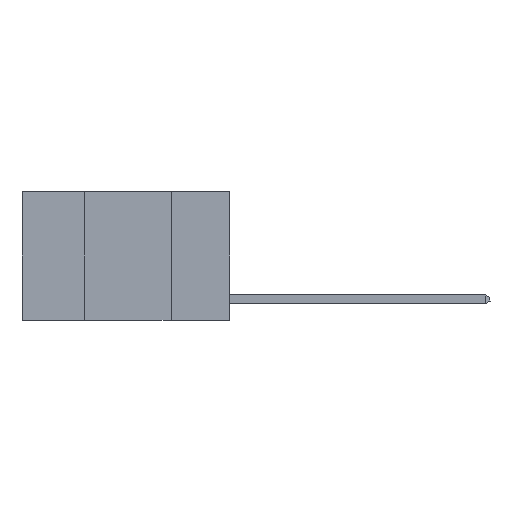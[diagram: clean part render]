
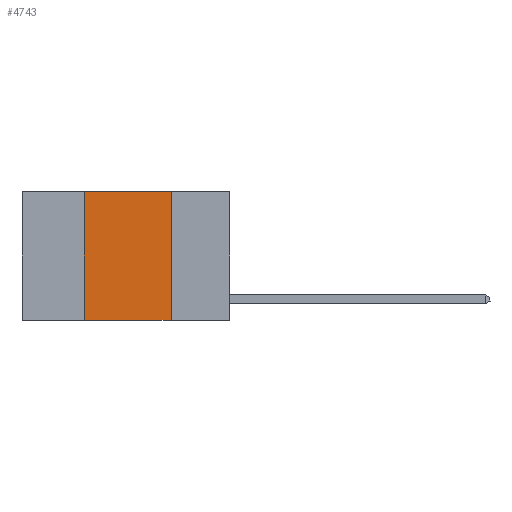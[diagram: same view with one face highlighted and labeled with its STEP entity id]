
A CAD part, left-side view. The second image highlights one B-rep face of the part: STEP entity #4743.
In plain terms, the highlighted planar face has unit normal (-1, 0, 0).
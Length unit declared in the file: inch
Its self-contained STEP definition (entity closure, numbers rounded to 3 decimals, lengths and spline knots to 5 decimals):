
#168 = PLANE ( 'NONE',  #10756 ) ;
#382 = DIRECTION ( 'NONE',  ( 0., 0., -1. ) ) ;
#2377 = ORIENTED_EDGE ( 'NONE', *, *, #10559, .F. ) ;
#3286 = VERTEX_POINT ( 'NONE', #4588 ) ;
#4561 = LINE ( 'NONE', #10851, #15903 ) ;
#4588 = CARTESIAN_POINT ( 'NONE',  ( 0., 0.17, -0.37 ) ) ;
#4635 = CARTESIAN_POINT ( 'NONE',  ( 0., 0.17, 0. ) ) ;
#4743 = ADVANCED_FACE ( 'NONE', ( #15711 ), #168, .F. ) ;
#7026 = EDGE_CURVE ( 'NONE', #7331, #3286, #4561, .T. ) ;
#7036 = LINE ( 'NONE', #19279, #10095 ) ;
#7270 = VERTEX_POINT ( 'NONE', #19467 ) ;
#7331 = VERTEX_POINT ( 'NONE', #8660 ) ;
#8660 = CARTESIAN_POINT ( 'NONE',  ( 0., 0.42, -0.37 ) ) ;
#9662 = ORIENTED_EDGE ( 'NONE', *, *, #11204, .F. ) ;
#10020 = CARTESIAN_POINT ( 'NONE',  ( 0., 0.42, 0. ) ) ;
#10095 = VECTOR ( 'NONE', #19478, 39.37008 ) ;
#10559 = EDGE_CURVE ( 'NONE', #18248, #7270, #7036, .T. ) ;
#10756 = AXIS2_PLACEMENT_3D ( 'NONE', #19101, #14469, #382 ) ;
#10851 = CARTESIAN_POINT ( 'NONE',  ( 0., 0.6, -0.37 ) ) ;
#11204 = EDGE_CURVE ( 'NONE', #7270, #3286, #18518, .T. ) ;
#11758 = VECTOR ( 'NONE', #18741, 39.37008 ) ;
#12166 = LINE ( 'NONE', #12579, #18736 ) ;
#12579 = CARTESIAN_POINT ( 'NONE',  ( 0., 0.42, 0. ) ) ;
#14469 = DIRECTION ( 'NONE',  ( 1., 0., 0. ) ) ;
#15502 = ORIENTED_EDGE ( 'NONE', *, *, #20222, .F. ) ;
#15711 = FACE_OUTER_BOUND ( 'NONE', #17831, .T. ) ;
#15903 = VECTOR ( 'NONE', #18776, 39.37008 ) ;
#16183 = ORIENTED_EDGE ( 'NONE', *, *, #7026, .T. ) ;
#17288 = DIRECTION ( 'NONE',  ( 0., 0., 1. ) ) ;
#17831 = EDGE_LOOP ( 'NONE', ( #9662, #2377, #15502, #16183 ) ) ;
#18248 = VERTEX_POINT ( 'NONE', #10020 ) ;
#18518 = LINE ( 'NONE', #4635, #11758 ) ;
#18736 = VECTOR ( 'NONE', #17288, 39.37008 ) ;
#18741 = DIRECTION ( 'NONE',  ( 0., 0., -1. ) ) ;
#18776 = DIRECTION ( 'NONE',  ( 0., -1., 0. ) ) ;
#19101 = CARTESIAN_POINT ( 'NONE',  ( 0., 0.6, 0. ) ) ;
#19279 = CARTESIAN_POINT ( 'NONE',  ( 0., 0.6, 0. ) ) ;
#19467 = CARTESIAN_POINT ( 'NONE',  ( 0., 0.17, 0. ) ) ;
#19478 = DIRECTION ( 'NONE',  ( 0., -1., 0. ) ) ;
#20222 = EDGE_CURVE ( 'NONE', #7331, #18248, #12166, .T. ) ;
